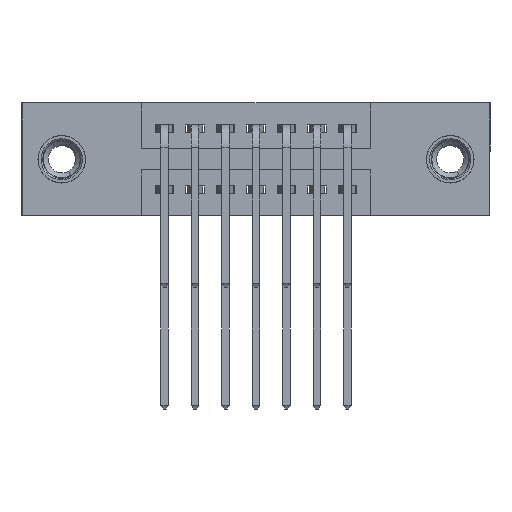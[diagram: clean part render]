
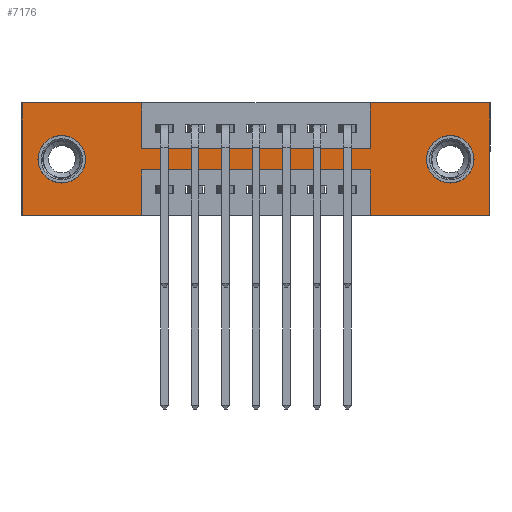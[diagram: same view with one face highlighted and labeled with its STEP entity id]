
A CAD part, front view. The second image highlights one B-rep face of the part: STEP entity #7176.
In plain terms, the highlighted planar face has unit normal (0, -1, 0).
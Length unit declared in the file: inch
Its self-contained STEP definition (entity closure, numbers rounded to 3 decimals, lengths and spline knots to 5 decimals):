
#34 = CARTESIAN_POINT ( 'NONE',  ( 1.535, 0., 0. ) ) ;
#154 = DIRECTION ( 'NONE',  ( 0., 0., 1. ) ) ;
#317 = CARTESIAN_POINT ( 'NONE',  ( 0.3925, 0., 0. ) ) ;
#335 = CARTESIAN_POINT ( 'NONE',  ( 0., 0., -0.37 ) ) ;
#394 = CARTESIAN_POINT ( 'NONE',  ( 0.3925, 0., -0.37 ) ) ;
#443 = EDGE_CURVE ( 'NONE', #13970, #4506, #2210, .T. ) ;
#555 = AXIS2_PLACEMENT_3D ( 'NONE', #12345, #5804, #9093 ) ;
#720 = CARTESIAN_POINT ( 'NONE',  ( 0., 0., 0. ) ) ;
#755 = CARTESIAN_POINT ( 'NONE',  ( 1.1425, 0., -0.22 ) ) ;
#767 = ORIENTED_EDGE ( 'NONE', *, *, #3303, .F. ) ;
#769 = EDGE_CURVE ( 'NONE', #779, #8801, #1192, .T. ) ;
#779 = VERTEX_POINT ( 'NONE', #3651 ) ;
#1049 = CARTESIAN_POINT ( 'NONE',  ( 1.535, 0., -0.37 ) ) ;
#1077 = LINE ( 'NONE', #4917, #7877 ) ;
#1192 = CIRCLE ( 'NONE', #555, 0.078 ) ;
#1518 = LINE ( 'NONE', #2082, #7145 ) ;
#1657 = VERTEX_POINT ( 'NONE', #755 ) ;
#1938 = CARTESIAN_POINT ( 'NONE',  ( 1.1425, 0., -0.37 ) ) ;
#2082 = CARTESIAN_POINT ( 'NONE',  ( 0., 0., -0.37 ) ) ;
#2165 = DIRECTION ( 'NONE',  ( 0., 1., 0. ) ) ;
#2210 = CIRCLE ( 'NONE', #10647, 0.078 ) ;
#2221 = EDGE_CURVE ( 'NONE', #7499, #11258, #8823, .T. ) ;
#2268 = VERTEX_POINT ( 'NONE', #10595 ) ;
#2349 = DIRECTION ( 'NONE',  ( 1., 0., 0. ) ) ;
#2363 = VERTEX_POINT ( 'NONE', #1938 ) ;
#2439 = EDGE_CURVE ( 'NONE', #1657, #4474, #7248, .T. ) ;
#2705 = EDGE_CURVE ( 'NONE', #10194, #10395, #5867, .T. ) ;
#2839 = EDGE_CURVE ( 'NONE', #4474, #7972, #5491, .T. ) ;
#2924 = DIRECTION ( 'NONE',  ( 0., -1., 0. ) ) ;
#2986 = VECTOR ( 'NONE', #13653, 39.37008 ) ;
#3108 = ORIENTED_EDGE ( 'NONE', *, *, #8515, .F. ) ;
#3201 = CARTESIAN_POINT ( 'NONE',  ( 0.3925, 0., -0.37 ) ) ;
#3303 = EDGE_CURVE ( 'NONE', #7972, #7499, #1518, .T. ) ;
#3421 = DIRECTION ( 'NONE',  ( 0., 0., -1. ) ) ;
#3528 = DIRECTION ( 'NONE',  ( 0., 0., -1. ) ) ;
#3562 = EDGE_LOOP ( 'NONE', ( #10836, #13686, #5992, #11977, #3108, #10626, #5475, #9843, #10907, #10164, #6659, #767 ) ) ;
#3651 = CARTESIAN_POINT ( 'NONE',  ( 1.405, 0., -0.263 ) ) ;
#3803 = ORIENTED_EDGE ( 'NONE', *, *, #10808, .T. ) ;
#3832 = AXIS2_PLACEMENT_3D ( 'NONE', #13883, #2924, #11671 ) ;
#3861 = VECTOR ( 'NONE', #11705, 39.37008 ) ;
#4076 = DIRECTION ( 'NONE',  ( 1., 0., 0. ) ) ;
#4474 = VERTEX_POINT ( 'NONE', #12741 ) ;
#4501 = CARTESIAN_POINT ( 'NONE',  ( 0.3925, 0., 0. ) ) ;
#4506 = VERTEX_POINT ( 'NONE', #8924 ) ;
#4596 = EDGE_CURVE ( 'NONE', #2268, #11778, #8665, .T. ) ;
#4758 = DIRECTION ( 'NONE',  ( 0., 0., 1. ) ) ;
#4917 = CARTESIAN_POINT ( 'NONE',  ( 0., 0., 0. ) ) ;
#5264 = DIRECTION ( 'NONE',  ( 0., 1., 0. ) ) ;
#5475 = ORIENTED_EDGE ( 'NONE', *, *, #4596, .F. ) ;
#5491 = LINE ( 'NONE', #394, #9785 ) ;
#5622 = CARTESIAN_POINT ( 'NONE',  ( 0.3925, 0., -0.15 ) ) ;
#5763 = VECTOR ( 'NONE', #4758, 39.37008 ) ;
#5804 = DIRECTION ( 'NONE',  ( 0., 1., 0. ) ) ;
#5867 = LINE ( 'NONE', #4501, #6546 ) ;
#5923 = ORIENTED_EDGE ( 'NONE', *, *, #769, .T. ) ;
#5992 = ORIENTED_EDGE ( 'NONE', *, *, #12469, .F. ) ;
#6049 = CARTESIAN_POINT ( 'NONE',  ( 0., 0., 0. ) ) ;
#6241 = CARTESIAN_POINT ( 'NONE',  ( 1.405, 0., -0.185 ) ) ;
#6546 = VECTOR ( 'NONE', #3421, 39.37008 ) ;
#6659 = ORIENTED_EDGE ( 'NONE', *, *, #2221, .F. ) ;
#6850 = EDGE_LOOP ( 'NONE', ( #3803, #5923 ) ) ;
#6935 = LINE ( 'NONE', #720, #3861 ) ;
#7145 = VECTOR ( 'NONE', #10003, 39.37008 ) ;
#7176 = ADVANCED_FACE ( 'NONE', ( #12451, #8859, #8164 ), #9488, .T. ) ;
#7248 = LINE ( 'NONE', #7740, #9484 ) ;
#7429 = LINE ( 'NONE', #335, #11543 ) ;
#7499 = VERTEX_POINT ( 'NONE', #9215 ) ;
#7516 = DIRECTION ( 'NONE',  ( 0., 0., 1. ) ) ;
#7740 = CARTESIAN_POINT ( 'NONE',  ( 0.3925, 0., -0.22 ) ) ;
#7767 = EDGE_CURVE ( 'NONE', #4506, #13970, #12420, .T. ) ;
#7825 = CARTESIAN_POINT ( 'NONE',  ( 1.535, 0., 0. ) ) ;
#7877 = VECTOR ( 'NONE', #4076, 39.37008 ) ;
#7972 = VERTEX_POINT ( 'NONE', #3201 ) ;
#8130 = CARTESIAN_POINT ( 'NONE',  ( 1.1425, 0., 0. ) ) ;
#8164 = FACE_OUTER_BOUND ( 'NONE', #3562, .T. ) ;
#8372 = CARTESIAN_POINT ( 'NONE',  ( 0., 0., 0. ) ) ;
#8434 = EDGE_CURVE ( 'NONE', #11149, #2363, #7429, .T. ) ;
#8486 = LINE ( 'NONE', #9354, #13914 ) ;
#8515 = EDGE_CURVE ( 'NONE', #11195, #11149, #12111, .T. ) ;
#8665 = LINE ( 'NONE', #9260, #5763 ) ;
#8693 = CARTESIAN_POINT ( 'NONE',  ( 0.13, 0., -0.185 ) ) ;
#8724 = VECTOR ( 'NONE', #2349, 39.37008 ) ;
#8801 = VERTEX_POINT ( 'NONE', #10026 ) ;
#8823 = LINE ( 'NONE', #6049, #2986 ) ;
#8859 = FACE_BOUND ( 'NONE', #11794, .T. ) ;
#8924 = CARTESIAN_POINT ( 'NONE',  ( 0.13, 0., -0.107 ) ) ;
#9093 = DIRECTION ( 'NONE',  ( 0., 0., -1. ) ) ;
#9215 = CARTESIAN_POINT ( 'NONE',  ( 0., 0., -0.37 ) ) ;
#9243 = LINE ( 'NONE', #9905, #8724 ) ;
#9260 = CARTESIAN_POINT ( 'NONE',  ( 1.1425, 0., 0. ) ) ;
#9310 = DIRECTION ( 'NONE',  ( 0., 1., 0. ) ) ;
#9354 = CARTESIAN_POINT ( 'NONE',  ( 1.1425, 0., -0.37 ) ) ;
#9484 = VECTOR ( 'NONE', #10849, 39.37008 ) ;
#9488 = PLANE ( 'NONE',  #3832 ) ;
#9624 = CARTESIAN_POINT ( 'NONE',  ( 0.13, 0., -0.263 ) ) ;
#9785 = VECTOR ( 'NONE', #3528, 39.37008 ) ;
#9786 = ORIENTED_EDGE ( 'NONE', *, *, #7767, .T. ) ;
#9843 = ORIENTED_EDGE ( 'NONE', *, *, #10331, .F. ) ;
#9905 = CARTESIAN_POINT ( 'NONE',  ( 0.3925, 0., -0.15 ) ) ;
#10003 = DIRECTION ( 'NONE',  ( -1., 0., 0. ) ) ;
#10012 = EDGE_CURVE ( 'NONE', #11258, #10194, #1077, .T. ) ;
#10026 = CARTESIAN_POINT ( 'NONE',  ( 1.405, 0., -0.107 ) ) ;
#10081 = VECTOR ( 'NONE', #11067, 39.37008 ) ;
#10164 = ORIENTED_EDGE ( 'NONE', *, *, #10012, .F. ) ;
#10175 = DIRECTION ( 'NONE',  ( -1., 0., 0. ) ) ;
#10194 = VERTEX_POINT ( 'NONE', #317 ) ;
#10331 = EDGE_CURVE ( 'NONE', #10395, #2268, #9243, .T. ) ;
#10395 = VERTEX_POINT ( 'NONE', #5622 ) ;
#10460 = DIRECTION ( 'NONE',  ( 0., 0., 1. ) ) ;
#10595 = CARTESIAN_POINT ( 'NONE',  ( 1.1425, 0., -0.15 ) ) ;
#10626 = ORIENTED_EDGE ( 'NONE', *, *, #12719, .F. ) ;
#10647 = AXIS2_PLACEMENT_3D ( 'NONE', #11968, #5264, #7516 ) ;
#10808 = EDGE_CURVE ( 'NONE', #8801, #779, #13622, .T. ) ;
#10836 = ORIENTED_EDGE ( 'NONE', *, *, #2839, .F. ) ;
#10849 = DIRECTION ( 'NONE',  ( -1., 0., 0. ) ) ;
#10907 = ORIENTED_EDGE ( 'NONE', *, *, #2705, .F. ) ;
#11067 = DIRECTION ( 'NONE',  ( 0., 0., -1. ) ) ;
#11149 = VERTEX_POINT ( 'NONE', #1049 ) ;
#11195 = VERTEX_POINT ( 'NONE', #34 ) ;
#11258 = VERTEX_POINT ( 'NONE', #8372 ) ;
#11542 = DIRECTION ( 'NONE',  ( 0., 0., -1. ) ) ;
#11543 = VECTOR ( 'NONE', #10175, 39.37008 ) ;
#11671 = DIRECTION ( 'NONE',  ( 0., 0., -1. ) ) ;
#11705 = DIRECTION ( 'NONE',  ( 1., 0., 0. ) ) ;
#11778 = VERTEX_POINT ( 'NONE', #8130 ) ;
#11794 = EDGE_LOOP ( 'NONE', ( #9786, #12302 ) ) ;
#11968 = CARTESIAN_POINT ( 'NONE',  ( 0.13, 0., -0.185 ) ) ;
#11977 = ORIENTED_EDGE ( 'NONE', *, *, #8434, .F. ) ;
#12111 = LINE ( 'NONE', #7825, #10081 ) ;
#12265 = AXIS2_PLACEMENT_3D ( 'NONE', #8693, #2165, #154 ) ;
#12302 = ORIENTED_EDGE ( 'NONE', *, *, #443, .T. ) ;
#12345 = CARTESIAN_POINT ( 'NONE',  ( 1.405, 0., -0.185 ) ) ;
#12420 = CIRCLE ( 'NONE', #12265, 0.078 ) ;
#12451 = FACE_BOUND ( 'NONE', #6850, .T. ) ;
#12469 = EDGE_CURVE ( 'NONE', #2363, #1657, #8486, .T. ) ;
#12719 = EDGE_CURVE ( 'NONE', #11778, #11195, #6935, .T. ) ;
#12741 = CARTESIAN_POINT ( 'NONE',  ( 0.3925, 0., -0.22 ) ) ;
#12968 = AXIS2_PLACEMENT_3D ( 'NONE', #6241, #9310, #11542 ) ;
#13622 = CIRCLE ( 'NONE', #12968, 0.078 ) ;
#13653 = DIRECTION ( 'NONE',  ( 0., 0., 1. ) ) ;
#13686 = ORIENTED_EDGE ( 'NONE', *, *, #2439, .F. ) ;
#13883 = CARTESIAN_POINT ( 'NONE',  ( 0., 0., -0.37 ) ) ;
#13914 = VECTOR ( 'NONE', #10460, 39.37008 ) ;
#13970 = VERTEX_POINT ( 'NONE', #9624 ) ;
